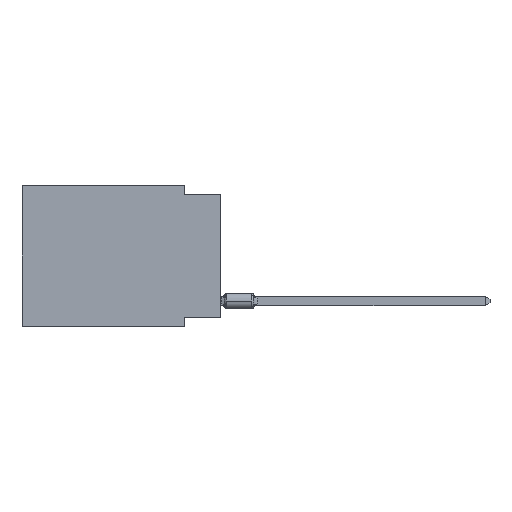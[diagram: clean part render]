
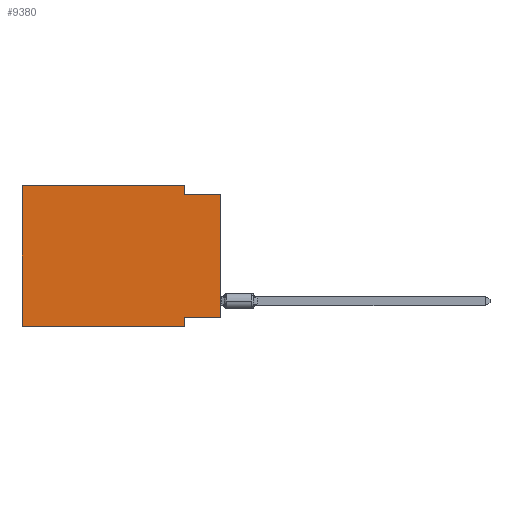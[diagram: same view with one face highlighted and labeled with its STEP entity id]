
A CAD part, left-side view. The second image highlights one B-rep face of the part: STEP entity #9380.
In plain terms, the highlighted planar face has unit normal (-1, 0, 0).
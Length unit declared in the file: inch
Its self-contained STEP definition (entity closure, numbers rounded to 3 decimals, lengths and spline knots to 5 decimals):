
#1745 = CARTESIAN_POINT ( 'NONE',  ( 0., 0.1, 0. ) ) ;
#2075 = CARTESIAN_POINT ( 'NONE',  ( 0., 0.1, -0.39 ) ) ;
#2562 = FACE_OUTER_BOUND ( 'NONE', #9921, .T. ) ;
#3038 = CARTESIAN_POINT ( 'NONE',  ( 0., 0., -0.025 ) ) ;
#5172 = EDGE_CURVE ( 'NONE', #28275, #37137, #46630, .T. ) ;
#5417 = CARTESIAN_POINT ( 'NONE',  ( 0., 0.55, -0.39 ) ) ;
#5508 = VERTEX_POINT ( 'NONE', #5417 ) ;
#6458 = CARTESIAN_POINT ( 'NONE',  ( 0., 0.55, 0. ) ) ;
#7193 = DIRECTION ( 'NONE',  ( 0., 0., -1. ) ) ;
#7413 = LINE ( 'NONE', #44160, #39345 ) ;
#8049 = CARTESIAN_POINT ( 'NONE',  ( 0., 0., -0.025 ) ) ;
#9082 = LINE ( 'NONE', #1745, #32097 ) ;
#9380 = ADVANCED_FACE ( 'NONE', ( #2562 ), #17500, .F. ) ;
#9763 = DIRECTION ( 'NONE',  ( 0., -1., 0. ) ) ;
#9921 = EDGE_LOOP ( 'NONE', ( #23277, #46369, #25581, #10775, #13002, #37512, #37413, #13834 ) ) ;
#10637 = DIRECTION ( 'NONE',  ( 1., 0., 0. ) ) ;
#10775 = ORIENTED_EDGE ( 'NONE', *, *, #43505, .F. ) ;
#11755 = EDGE_CURVE ( 'NONE', #17379, #38553, #18479, .T. ) ;
#13002 = ORIENTED_EDGE ( 'NONE', *, *, #18815, .F. ) ;
#13382 = VECTOR ( 'NONE', #45962, 39.37008 ) ;
#13705 = CARTESIAN_POINT ( 'NONE',  ( 0., 0.1, -0.39 ) ) ;
#13834 = ORIENTED_EDGE ( 'NONE', *, *, #45287, .F. ) ;
#13935 = CARTESIAN_POINT ( 'NONE',  ( 0., 0.55, 0. ) ) ;
#14050 = DIRECTION ( 'NONE',  ( 0., -1., 0. ) ) ;
#15477 = EDGE_CURVE ( 'NONE', #34697, #17379, #9082, .T. ) ;
#15896 = LINE ( 'NONE', #30567, #30431 ) ;
#17379 = VERTEX_POINT ( 'NONE', #33757 ) ;
#17500 = PLANE ( 'NONE',  #47250 ) ;
#18159 = CARTESIAN_POINT ( 'NONE',  ( 0., 0.55, 0. ) ) ;
#18479 = LINE ( 'NONE', #3038, #34993 ) ;
#18815 = EDGE_CURVE ( 'NONE', #5508, #36105, #28635, .T. ) ;
#19198 = CARTESIAN_POINT ( 'NONE',  ( 0., 0.1, -0.365 ) ) ;
#20795 = LINE ( 'NONE', #27656, #31301 ) ;
#22711 = VERTEX_POINT ( 'NONE', #42322 ) ;
#23277 = ORIENTED_EDGE ( 'NONE', *, *, #37380, .T. ) ;
#24399 = VECTOR ( 'NONE', #39544, 39.37008 ) ;
#24812 = EDGE_CURVE ( 'NONE', #5508, #37137, #20795, .T. ) ;
#25581 = ORIENTED_EDGE ( 'NONE', *, *, #15477, .F. ) ;
#27131 = CARTESIAN_POINT ( 'NONE',  ( 0., 0., -0.365 ) ) ;
#27656 = CARTESIAN_POINT ( 'NONE',  ( 0., 0.55, -0.39 ) ) ;
#28275 = VERTEX_POINT ( 'NONE', #19198 ) ;
#28635 = LINE ( 'NONE', #13935, #42385 ) ;
#30431 = VECTOR ( 'NONE', #41130, 39.37008 ) ;
#30567 = CARTESIAN_POINT ( 'NONE',  ( 0., 0., 0. ) ) ;
#31301 = VECTOR ( 'NONE', #9763, 39.37008 ) ;
#32097 = VECTOR ( 'NONE', #34173, 39.37008 ) ;
#32298 = DIRECTION ( 'NONE',  ( 0., 0., 1. ) ) ;
#33757 = CARTESIAN_POINT ( 'NONE',  ( 0., 0.1, -0.025 ) ) ;
#34173 = DIRECTION ( 'NONE',  ( 0., 0., -1. ) ) ;
#34697 = VERTEX_POINT ( 'NONE', #38255 ) ;
#34993 = VECTOR ( 'NONE', #14050, 39.37008 ) ;
#36105 = VERTEX_POINT ( 'NONE', #18159 ) ;
#37137 = VERTEX_POINT ( 'NONE', #13705 ) ;
#37380 = EDGE_CURVE ( 'NONE', #22711, #38553, #15896, .T. ) ;
#37413 = ORIENTED_EDGE ( 'NONE', *, *, #5172, .F. ) ;
#37512 = ORIENTED_EDGE ( 'NONE', *, *, #24812, .T. ) ;
#38255 = CARTESIAN_POINT ( 'NONE',  ( 0., 0.1, 0. ) ) ;
#38553 = VERTEX_POINT ( 'NONE', #8049 ) ;
#39097 = LINE ( 'NONE', #27131, #13382 ) ;
#39345 = VECTOR ( 'NONE', #41443, 39.37008 ) ;
#39544 = DIRECTION ( 'NONE',  ( 0., 0., -1. ) ) ;
#41130 = DIRECTION ( 'NONE',  ( 0., 0., 1. ) ) ;
#41443 = DIRECTION ( 'NONE',  ( 0., -1., 0. ) ) ;
#42322 = CARTESIAN_POINT ( 'NONE',  ( 0., 0., -0.365 ) ) ;
#42385 = VECTOR ( 'NONE', #32298, 39.37008 ) ;
#43505 = EDGE_CURVE ( 'NONE', #36105, #34697, #7413, .T. ) ;
#44160 = CARTESIAN_POINT ( 'NONE',  ( 0., 0.55, 0. ) ) ;
#45287 = EDGE_CURVE ( 'NONE', #22711, #28275, #39097, .T. ) ;
#45962 = DIRECTION ( 'NONE',  ( 0., 1., 0. ) ) ;
#46369 = ORIENTED_EDGE ( 'NONE', *, *, #11755, .F. ) ;
#46630 = LINE ( 'NONE', #2075, #24399 ) ;
#47250 = AXIS2_PLACEMENT_3D ( 'NONE', #6458, #10637, #7193 ) ;
